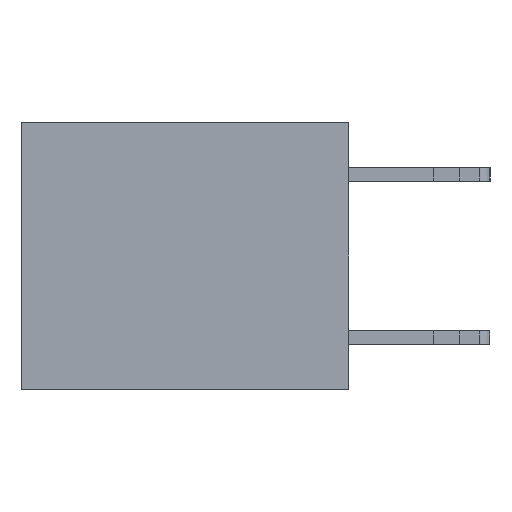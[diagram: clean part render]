
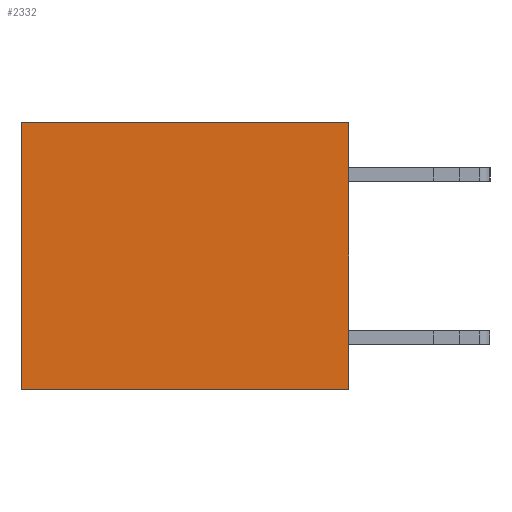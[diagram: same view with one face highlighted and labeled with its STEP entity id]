
A CAD part, left-side view. The second image highlights one B-rep face of the part: STEP entity #2332.
In plain terms, the highlighted planar face has unit normal (-1, 0, 0).
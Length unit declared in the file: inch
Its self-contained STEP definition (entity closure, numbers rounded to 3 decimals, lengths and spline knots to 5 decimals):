
#3 = VECTOR ( 'NONE', #12823, 39.37008 ) ;
#780 = VECTOR ( 'NONE', #4312, 39.37008 ) ;
#1864 = AXIS2_PLACEMENT_3D ( 'NONE', #13856, #15024, #13695 ) ;
#2332 = ADVANCED_FACE ( 'NONE', ( #14546 ), #11502, .F. ) ;
#2381 = VERTEX_POINT ( 'NONE', #12713 ) ;
#2965 = EDGE_CURVE ( 'NONE', #13890, #3387, #3982, .T. ) ;
#3387 = VERTEX_POINT ( 'NONE', #9629 ) ;
#3982 = LINE ( 'NONE', #13675, #13040 ) ;
#4312 = DIRECTION ( 'NONE',  ( 0., 0., -1. ) ) ;
#4763 = ORIENTED_EDGE ( 'NONE', *, *, #2965, .T. ) ;
#5452 = ORIENTED_EDGE ( 'NONE', *, *, #12424, .F. ) ;
#6347 = EDGE_CURVE ( 'NONE', #2381, #10714, #13097, .T. ) ;
#6870 = EDGE_CURVE ( 'NONE', #3387, #10714, #13813, .T. ) ;
#7183 = EDGE_LOOP ( 'NONE', ( #14069, #8781, #5452, #4763 ) ) ;
#7480 = DIRECTION ( 'NONE',  ( 0., 1., 0. ) ) ;
#8781 = ORIENTED_EDGE ( 'NONE', *, *, #6347, .F. ) ;
#9629 = CARTESIAN_POINT ( 'NONE',  ( 0.3165, 0.6, 0. ) ) ;
#10315 = CARTESIAN_POINT ( 'NONE',  ( 0.3165, 0., -0.49 ) ) ;
#10682 = CARTESIAN_POINT ( 'NONE',  ( 0.3165, 0., -0.49 ) ) ;
#10714 = VERTEX_POINT ( 'NONE', #11930 ) ;
#11502 = PLANE ( 'NONE',  #1864 ) ;
#11699 = CARTESIAN_POINT ( 'NONE',  ( 0.3165, 0.6, -0.49 ) ) ;
#11930 = CARTESIAN_POINT ( 'NONE',  ( 0.3165, 0.6, -0.49 ) ) ;
#12424 = EDGE_CURVE ( 'NONE', #13890, #2381, #13797, .T. ) ;
#12687 = VECTOR ( 'NONE', #15552, 39.37008 ) ;
#12713 = CARTESIAN_POINT ( 'NONE',  ( 0.3165, 0., -0.49 ) ) ;
#12823 = DIRECTION ( 'NONE',  ( 0., 1., 0. ) ) ;
#13040 = VECTOR ( 'NONE', #7480, 39.37008 ) ;
#13097 = LINE ( 'NONE', #10315, #3 ) ;
#13252 = CARTESIAN_POINT ( 'NONE',  ( 0.3165, 0., 0. ) ) ;
#13675 = CARTESIAN_POINT ( 'NONE',  ( 0.3165, 0., 0. ) ) ;
#13695 = DIRECTION ( 'NONE',  ( 0., 0., -1. ) ) ;
#13797 = LINE ( 'NONE', #10682, #12687 ) ;
#13813 = LINE ( 'NONE', #11699, #780 ) ;
#13856 = CARTESIAN_POINT ( 'NONE',  ( 0.3165, 0., -0.49 ) ) ;
#13890 = VERTEX_POINT ( 'NONE', #13252 ) ;
#14069 = ORIENTED_EDGE ( 'NONE', *, *, #6870, .T. ) ;
#14546 = FACE_OUTER_BOUND ( 'NONE', #7183, .T. ) ;
#15024 = DIRECTION ( 'NONE',  ( 1., 0., 0. ) ) ;
#15552 = DIRECTION ( 'NONE',  ( 0., 0., -1. ) ) ;
